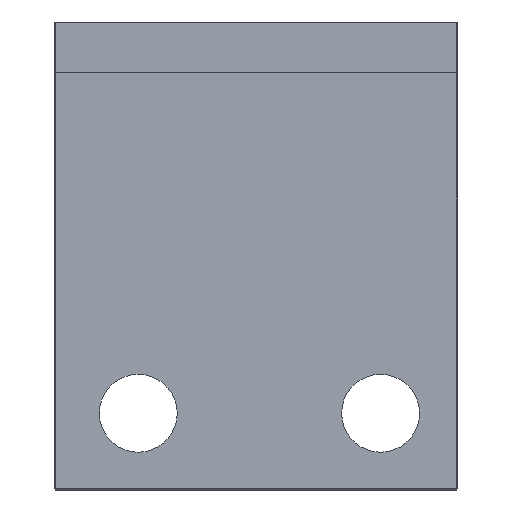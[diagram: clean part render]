
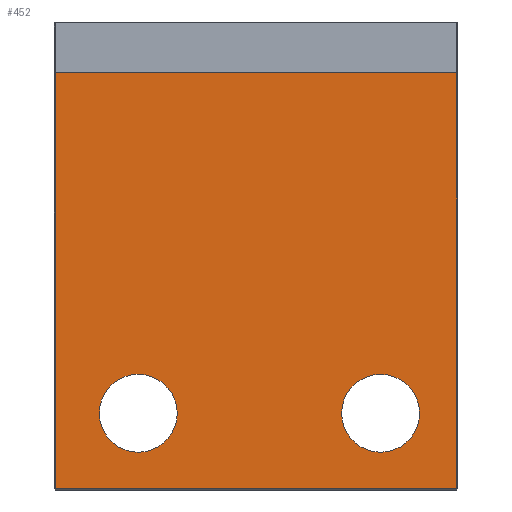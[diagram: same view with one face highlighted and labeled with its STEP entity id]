
A CAD part, front view. The second image highlights one B-rep face of the part: STEP entity #452.
In plain terms, the highlighted planar face has unit normal (0, -1, 0).
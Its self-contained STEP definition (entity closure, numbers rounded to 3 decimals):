
#17=FACE_BOUND('',#82,.T.);
#18=FACE_BOUND('',#83,.T.);
#23=CIRCLE('',#505,1.448);
#24=CIRCLE('',#507,1.448);
#53=FACE_OUTER_BOUND('',#81,.T.);
#81=EDGE_LOOP('',(#398,#399,#400,#401));
#82=EDGE_LOOP('',(#402));
#83=EDGE_LOOP('',(#403));
#110=LINE('',#693,#160);
#117=LINE('',#706,#167);
#120=LINE('',#712,#170);
#132=LINE('',#733,#182);
#160=VECTOR('',#561,10.);
#167=VECTOR('',#574,10.);
#170=VECTOR('',#581,10.);
#182=VECTOR('',#601,1000.);
#205=VERTEX_POINT('',#675);
#208=VERTEX_POINT('',#685);
#211=VERTEX_POINT('',#698);
#214=VERTEX_POINT('',#711);
#222=VERTEX_POINT('',#748);
#223=VERTEX_POINT('',#752);
#252=EDGE_CURVE('',#208,#205,#110,.T.);
#259=EDGE_CURVE('',#211,#208,#117,.T.);
#262=EDGE_CURVE('',#214,#211,#120,.T.);
#274=EDGE_CURVE('',#214,#205,#132,.T.);
#281=EDGE_CURVE('',#222,#222,#23,.F.);
#283=EDGE_CURVE('',#223,#223,#24,.F.);
#398=ORIENTED_EDGE('',*,*,#262,.F.);
#399=ORIENTED_EDGE('',*,*,#274,.T.);
#400=ORIENTED_EDGE('',*,*,#252,.F.);
#401=ORIENTED_EDGE('',*,*,#259,.F.);
#402=ORIENTED_EDGE('',*,*,#281,.T.);
#403=ORIENTED_EDGE('',*,*,#283,.T.);
#426=PLANE('',#508);
#452=ADVANCED_FACE('',(#53,#17,#18),#426,.F.);
#505=AXIS2_PLACEMENT_3D('',#750,#624,#625);
#507=AXIS2_PLACEMENT_3D('',#754,#629,#630);
#508=AXIS2_PLACEMENT_3D('',#755,#631,#632);
#561=DIRECTION('',(0.,0.,1.));
#574=DIRECTION('',(-1.,0.,0.));
#581=DIRECTION('',(0.,0.,-1.));
#601=DIRECTION('',(-1.,0.,0.));
#624=DIRECTION('center_axis',(0.,-1.,0.));
#625=DIRECTION('ref_axis',(0.,0.,-1.));
#629=DIRECTION('center_axis',(0.,-1.,0.));
#630=DIRECTION('ref_axis',(0.,0.,-1.));
#631=DIRECTION('center_axis',(0.,1.,0.));
#632=DIRECTION('ref_axis',(0.,0.,1.));
#675=CARTESIAN_POINT('',(0.05,-19.04,40.605));
#685=CARTESIAN_POINT('',(0.05,-19.04,25.155));
#693=CARTESIAN_POINT('',(0.05,-19.04,20.303));
#698=CARTESIAN_POINT('',(14.95,-19.04,25.155));
#706=CARTESIAN_POINT('',(15.,-19.04,25.155));
#711=CARTESIAN_POINT('',(14.95,-19.04,40.603));
#712=CARTESIAN_POINT('',(14.95,-19.04,20.303));
#733=CARTESIAN_POINT('',(15.,-19.04,40.603));
#748=CARTESIAN_POINT('',(3.127,-19.04,29.403));
#750=CARTESIAN_POINT('Origin',(3.127,-19.04,27.955));
#752=CARTESIAN_POINT('',(12.127,-19.04,29.403));
#754=CARTESIAN_POINT('Origin',(12.127,-19.04,27.955));
#755=CARTESIAN_POINT('Origin',(15.,-19.04,40.605));
